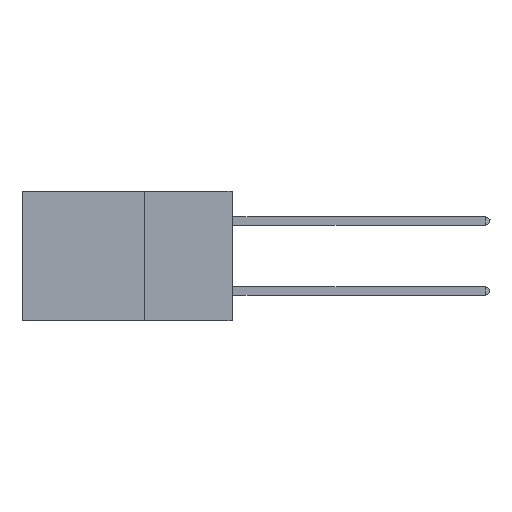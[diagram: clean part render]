
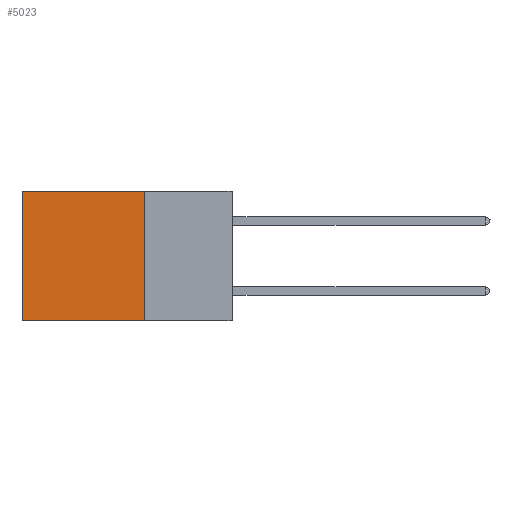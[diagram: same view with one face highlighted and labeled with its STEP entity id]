
A CAD part, left-side view. The second image highlights one B-rep face of the part: STEP entity #5023.
In plain terms, the highlighted planar face has unit normal (-1, 0, 0).
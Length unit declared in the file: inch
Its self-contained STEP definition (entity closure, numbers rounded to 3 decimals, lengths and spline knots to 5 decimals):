
#51 = DIRECTION ( 'NONE',  ( 0., 1., 0. ) ) ;
#86 = FACE_OUTER_BOUND ( 'NONE', #5535, .T. ) ;
#1033 = VECTOR ( 'NONE', #10039, 39.37008 ) ;
#1297 = CARTESIAN_POINT ( 'NONE',  ( 0.2875, 0.25, 0. ) ) ;
#1747 = CARTESIAN_POINT ( 'NONE',  ( 0.2875, 0.25, -0.37 ) ) ;
#2119 = VERTEX_POINT ( 'NONE', #2350 ) ;
#2170 = VECTOR ( 'NONE', #8175, 39.37008 ) ;
#2350 = CARTESIAN_POINT ( 'NONE',  ( 0.2875, 0.25, 0. ) ) ;
#2626 = CARTESIAN_POINT ( 'NONE',  ( 0.2875, 0.25, 0. ) ) ;
#3092 = LINE ( 'NONE', #1747, #16847 ) ;
#3864 = VERTEX_POINT ( 'NONE', #15660 ) ;
#3937 = VERTEX_POINT ( 'NONE', #10851 ) ;
#4141 = CARTESIAN_POINT ( 'NONE',  ( 0.2875, 0.6, 0. ) ) ;
#4447 = DIRECTION ( 'NONE',  ( 0., 0., -1. ) ) ;
#5023 = ADVANCED_FACE ( 'NONE', ( #86 ), #8386, .F. ) ;
#5535 = EDGE_LOOP ( 'NONE', ( #16233, #8390, #12154, #14468 ) ) ;
#7133 = EDGE_CURVE ( 'NONE', #3864, #7564, #3092, .T. ) ;
#7564 = VERTEX_POINT ( 'NONE', #15411 ) ;
#8087 = LINE ( 'NONE', #1297, #2170 ) ;
#8175 = DIRECTION ( 'NONE',  ( 0., 0., -1. ) ) ;
#8386 = PLANE ( 'NONE',  #16789 ) ;
#8390 = ORIENTED_EDGE ( 'NONE', *, *, #7133, .F. ) ;
#8566 = CARTESIAN_POINT ( 'NONE',  ( 0.2875, 0.25, 0. ) ) ;
#9673 = DIRECTION ( 'NONE',  ( 0., 1., 0. ) ) ;
#10039 = DIRECTION ( 'NONE',  ( 0., 0., -1. ) ) ;
#10851 = CARTESIAN_POINT ( 'NONE',  ( 0.2875, 0.6, 0. ) ) ;
#11304 = EDGE_CURVE ( 'NONE', #2119, #3937, #14837, .T. ) ;
#12154 = ORIENTED_EDGE ( 'NONE', *, *, #17215, .F. ) ;
#13819 = DIRECTION ( 'NONE',  ( 1., 0., 0. ) ) ;
#14468 = ORIENTED_EDGE ( 'NONE', *, *, #11304, .T. ) ;
#14837 = LINE ( 'NONE', #2626, #16899 ) ;
#15411 = CARTESIAN_POINT ( 'NONE',  ( 0.2875, 0.6, -0.37 ) ) ;
#15660 = CARTESIAN_POINT ( 'NONE',  ( 0.2875, 0.25, -0.37 ) ) ;
#16233 = ORIENTED_EDGE ( 'NONE', *, *, #17239, .T. ) ;
#16354 = LINE ( 'NONE', #4141, #1033 ) ;
#16789 = AXIS2_PLACEMENT_3D ( 'NONE', #8566, #13819, #4447 ) ;
#16847 = VECTOR ( 'NONE', #51, 39.37008 ) ;
#16899 = VECTOR ( 'NONE', #9673, 39.37008 ) ;
#17215 = EDGE_CURVE ( 'NONE', #2119, #3864, #8087, .T. ) ;
#17239 = EDGE_CURVE ( 'NONE', #3937, #7564, #16354, .T. ) ;
